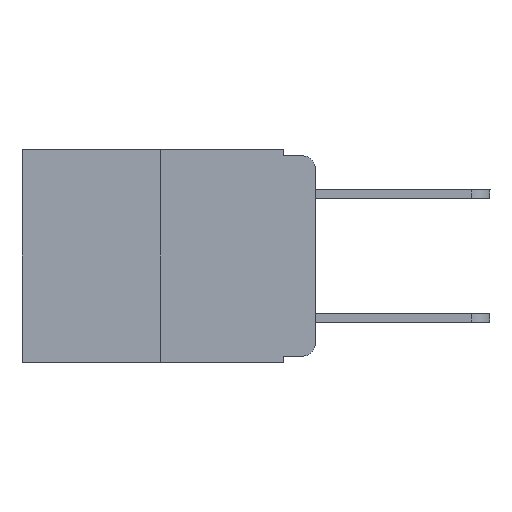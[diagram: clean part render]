
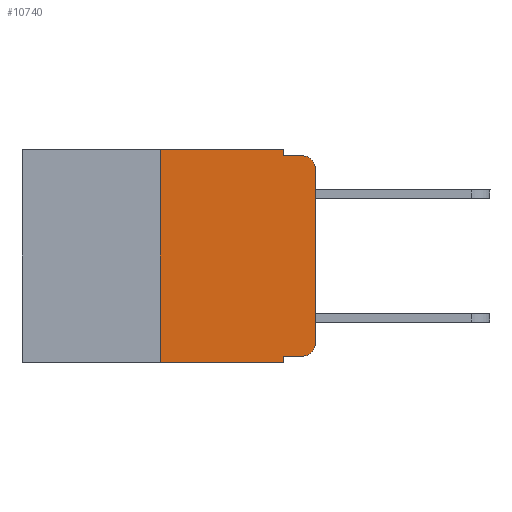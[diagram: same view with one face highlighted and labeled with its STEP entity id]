
A CAD part, left-side view. The second image highlights one B-rep face of the part: STEP entity #10740.
In plain terms, the highlighted planar face has unit normal (-1, 0, 0).
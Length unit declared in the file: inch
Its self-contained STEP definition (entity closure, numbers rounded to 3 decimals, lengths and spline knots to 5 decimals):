
#202 = VECTOR ( 'NONE', #5474, 39.37008 ) ;
#550 = VERTEX_POINT ( 'NONE', #8237 ) ;
#714 = CARTESIAN_POINT ( 'NONE',  ( 0., 0.25, 0. ) ) ;
#1132 = VERTEX_POINT ( 'NONE', #14878 ) ;
#1269 = CARTESIAN_POINT ( 'NONE',  ( 0., 0.051, 0. ) ) ;
#1274 = VECTOR ( 'NONE', #8893, 39.37008 ) ;
#1426 = ORIENTED_EDGE ( 'NONE', *, *, #17377, .F. ) ;
#2335 = LINE ( 'NONE', #714, #3568 ) ;
#2539 = LINE ( 'NONE', #20956, #19837 ) ;
#3073 = AXIS2_PLACEMENT_3D ( 'NONE', #10866, #5215, #16639 ) ;
#3101 = VERTEX_POINT ( 'NONE', #7868 ) ;
#3216 = VERTEX_POINT ( 'NONE', #8209 ) ;
#3334 = LINE ( 'NONE', #3529, #11802 ) ;
#3529 = CARTESIAN_POINT ( 'NONE',  ( 0., 0.051, -0.01 ) ) ;
#3568 = VECTOR ( 'NONE', #18160, 39.37008 ) ;
#4130 = CARTESIAN_POINT ( 'NONE',  ( 0., 0.051, -0.333 ) ) ;
#5051 = CARTESIAN_POINT ( 'NONE',  ( 0., 0.473, -0.343 ) ) ;
#5097 = LINE ( 'NONE', #4130, #6022 ) ;
#5208 = VERTEX_POINT ( 'NONE', #16767 ) ;
#5215 = DIRECTION ( 'NONE',  ( -1., 0., 0. ) ) ;
#5474 = DIRECTION ( 'NONE',  ( 0., -1., 0. ) ) ;
#5642 = DIRECTION ( 'NONE',  ( 0., 0., -1. ) ) ;
#5945 = PLANE ( 'NONE',  #12033 ) ;
#6022 = VECTOR ( 'NONE', #9961, 39.37008 ) ;
#6464 = LINE ( 'NONE', #1269, #1274 ) ;
#6770 = VERTEX_POINT ( 'NONE', #7329 ) ;
#7329 = CARTESIAN_POINT ( 'NONE',  ( 0., 0.25, 0. ) ) ;
#7794 = DIRECTION ( 'NONE',  ( -1., 0., 0. ) ) ;
#7868 = CARTESIAN_POINT ( 'NONE',  ( 0., 0.02, -0.333 ) ) ;
#7870 = DIRECTION ( 'NONE',  ( 1., 0., 0. ) ) ;
#7920 = EDGE_CURVE ( 'NONE', #550, #6770, #2335, .T. ) ;
#8209 = CARTESIAN_POINT ( 'NONE',  ( 0., 0., -0.313 ) ) ;
#8237 = CARTESIAN_POINT ( 'NONE',  ( 0., 0.25, -0.343 ) ) ;
#8360 = LINE ( 'NONE', #19815, #24396 ) ;
#8893 = DIRECTION ( 'NONE',  ( 0., 0., -1. ) ) ;
#9016 = DIRECTION ( 'NONE',  ( 0., -1., 0. ) ) ;
#9115 = CARTESIAN_POINT ( 'NONE',  ( 0., 0.051, -0.333 ) ) ;
#9427 = CARTESIAN_POINT ( 'NONE',  ( 0., 0.473, 0. ) ) ;
#9531 = VERTEX_POINT ( 'NONE', #17046 ) ;
#9961 = DIRECTION ( 'NONE',  ( 0., -1., 0. ) ) ;
#10519 = LINE ( 'NONE', #9427, #202 ) ;
#10534 = CARTESIAN_POINT ( 'NONE',  ( 0., 0.051, -0.343 ) ) ;
#10611 = LINE ( 'NONE', #5051, #14825 ) ;
#10740 = ADVANCED_FACE ( 'NONE', ( #21307 ), #5945, .F. ) ;
#10866 = CARTESIAN_POINT ( 'NONE',  ( 0., 0.02, -0.313 ) ) ;
#11487 = VERTEX_POINT ( 'NONE', #10534 ) ;
#11802 = VECTOR ( 'NONE', #15181, 39.37008 ) ;
#12033 = AXIS2_PLACEMENT_3D ( 'NONE', #13954, #7870, #23524 ) ;
#12095 = EDGE_LOOP ( 'NONE', ( #23846, #22993, #21378, #12537, #1426, #23987, #12223, #22349, #17342, #18122 ) ) ;
#12223 = ORIENTED_EDGE ( 'NONE', *, *, #14902, .T. ) ;
#12537 = ORIENTED_EDGE ( 'NONE', *, *, #12541, .F. ) ;
#12541 = EDGE_CURVE ( 'NONE', #1132, #5208, #2539, .T. ) ;
#13177 = CIRCLE ( 'NONE', #3073, 0.02 ) ;
#13638 = EDGE_CURVE ( 'NONE', #23417, #11487, #6464, .T. ) ;
#13954 = CARTESIAN_POINT ( 'NONE',  ( 0., 0.473, 0. ) ) ;
#14440 = CIRCLE ( 'NONE', #16679, 0.02 ) ;
#14825 = VECTOR ( 'NONE', #9016, 39.37008 ) ;
#14878 = CARTESIAN_POINT ( 'NONE',  ( 0., 0.051, 0. ) ) ;
#14902 = EDGE_CURVE ( 'NONE', #550, #11487, #10611, .T. ) ;
#15181 = DIRECTION ( 'NONE',  ( 0., -1., 0. ) ) ;
#15405 = DIRECTION ( 'NONE',  ( 0., 0., -1. ) ) ;
#16639 = DIRECTION ( 'NONE',  ( 0., 0., -1. ) ) ;
#16679 = AXIS2_PLACEMENT_3D ( 'NONE', #22940, #7794, #15405 ) ;
#16767 = CARTESIAN_POINT ( 'NONE',  ( 0., 0.051, -0.01 ) ) ;
#16963 = EDGE_CURVE ( 'NONE', #23417, #3101, #5097, .T. ) ;
#17046 = CARTESIAN_POINT ( 'NONE',  ( 0., 0., -0.03 ) ) ;
#17342 = ORIENTED_EDGE ( 'NONE', *, *, #16963, .T. ) ;
#17377 = EDGE_CURVE ( 'NONE', #6770, #1132, #10519, .T. ) ;
#17926 = DIRECTION ( 'NONE',  ( 0., 0., 1. ) ) ;
#18122 = ORIENTED_EDGE ( 'NONE', *, *, #21546, .T. ) ;
#18160 = DIRECTION ( 'NONE',  ( 0., 0., 1. ) ) ;
#19111 = EDGE_CURVE ( 'NONE', #5208, #24209, #3334, .T. ) ;
#19815 = CARTESIAN_POINT ( 'NONE',  ( 0., 0., 0. ) ) ;
#19837 = VECTOR ( 'NONE', #5642, 39.37008 ) ;
#20487 = EDGE_CURVE ( 'NONE', #9531, #24209, #14440, .T. ) ;
#20956 = CARTESIAN_POINT ( 'NONE',  ( 0., 0.051, 0. ) ) ;
#21307 = FACE_OUTER_BOUND ( 'NONE', #12095, .T. ) ;
#21378 = ORIENTED_EDGE ( 'NONE', *, *, #19111, .F. ) ;
#21546 = EDGE_CURVE ( 'NONE', #3101, #3216, #13177, .T. ) ;
#22349 = ORIENTED_EDGE ( 'NONE', *, *, #13638, .F. ) ;
#22940 = CARTESIAN_POINT ( 'NONE',  ( 0., 0.02, -0.03 ) ) ;
#22993 = ORIENTED_EDGE ( 'NONE', *, *, #20487, .T. ) ;
#23417 = VERTEX_POINT ( 'NONE', #9115 ) ;
#23524 = DIRECTION ( 'NONE',  ( 0., 0., -1. ) ) ;
#23846 = ORIENTED_EDGE ( 'NONE', *, *, #25057, .T. ) ;
#23987 = ORIENTED_EDGE ( 'NONE', *, *, #7920, .F. ) ;
#24209 = VERTEX_POINT ( 'NONE', #24404 ) ;
#24396 = VECTOR ( 'NONE', #17926, 39.37008 ) ;
#24404 = CARTESIAN_POINT ( 'NONE',  ( 0., 0.02, -0.01 ) ) ;
#25057 = EDGE_CURVE ( 'NONE', #3216, #9531, #8360, .T. ) ;
